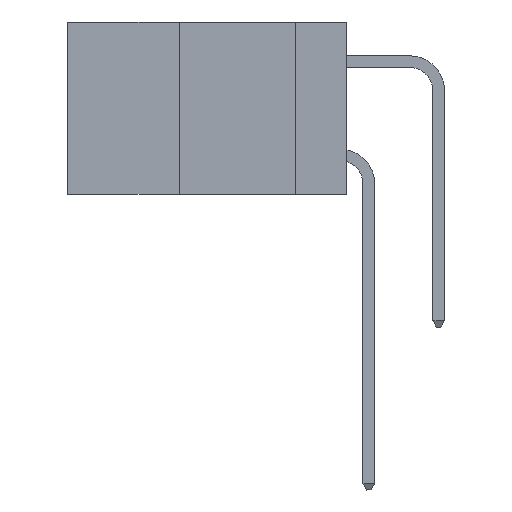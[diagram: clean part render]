
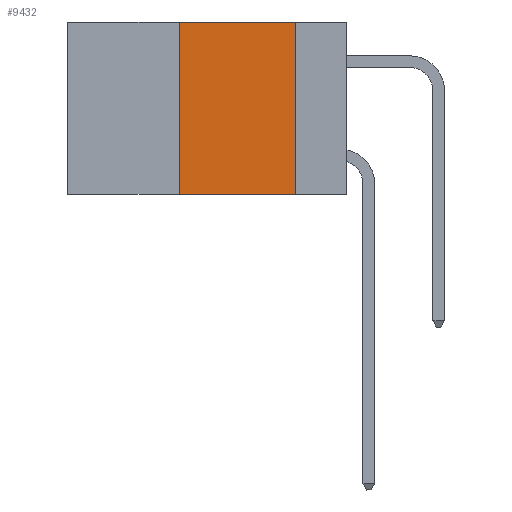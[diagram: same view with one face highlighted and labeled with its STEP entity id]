
A CAD part, left-side view. The second image highlights one B-rep face of the part: STEP entity #9432.
In plain terms, the highlighted planar face has unit normal (-1, 0, 0).
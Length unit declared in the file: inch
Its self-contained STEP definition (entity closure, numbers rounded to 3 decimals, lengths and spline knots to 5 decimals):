
#550 = LINE ( 'NONE', #8312, #8073 ) ;
#907 = ORIENTED_EDGE ( 'NONE', *, *, #11543, .F. ) ;
#1403 = LINE ( 'NONE', #4061, #6314 ) ;
#1874 = CARTESIAN_POINT ( 'NONE',  ( 0., 0.11, -0.37 ) ) ;
#1982 = CARTESIAN_POINT ( 'NONE',  ( 0., 0.36, -0.37 ) ) ;
#2194 = CARTESIAN_POINT ( 'NONE',  ( 0., 0.11, 0. ) ) ;
#2988 = LINE ( 'NONE', #5645, #7509 ) ;
#3065 = VERTEX_POINT ( 'NONE', #3408 ) ;
#3408 = CARTESIAN_POINT ( 'NONE',  ( 0., 0.36, 0. ) ) ;
#3437 = DIRECTION ( 'NONE',  ( 1., 0., 0. ) ) ;
#3936 = ORIENTED_EDGE ( 'NONE', *, *, #5729, .F. ) ;
#4061 = CARTESIAN_POINT ( 'NONE',  ( 0., 0.11, 0. ) ) ;
#4107 = DIRECTION ( 'NONE',  ( 0., 0., -1. ) ) ;
#4179 = LINE ( 'NONE', #4275, #7334 ) ;
#4275 = CARTESIAN_POINT ( 'NONE',  ( 0., 0.36, 0. ) ) ;
#4535 = EDGE_CURVE ( 'NONE', #11999, #9100, #2988, .T. ) ;
#4702 = ORIENTED_EDGE ( 'NONE', *, *, #4535, .T. ) ;
#5645 = CARTESIAN_POINT ( 'NONE',  ( 0., 0.6, -0.37 ) ) ;
#5729 = EDGE_CURVE ( 'NONE', #12109, #9100, #1403, .T. ) ;
#6010 = FACE_OUTER_BOUND ( 'NONE', #9294, .T. ) ;
#6205 = AXIS2_PLACEMENT_3D ( 'NONE', #8195, #3437, #10033 ) ;
#6314 = VECTOR ( 'NONE', #4107, 39.37008 ) ;
#6315 = PLANE ( 'NONE',  #6205 ) ;
#7334 = VECTOR ( 'NONE', #10843, 39.37008 ) ;
#7509 = VECTOR ( 'NONE', #11250, 39.37008 ) ;
#8073 = VECTOR ( 'NONE', #11093, 39.37008 ) ;
#8195 = CARTESIAN_POINT ( 'NONE',  ( 0., 0.6, 0. ) ) ;
#8312 = CARTESIAN_POINT ( 'NONE',  ( 0., 0.6, 0. ) ) ;
#8667 = ORIENTED_EDGE ( 'NONE', *, *, #10124, .F. ) ;
#9100 = VERTEX_POINT ( 'NONE', #1874 ) ;
#9294 = EDGE_LOOP ( 'NONE', ( #3936, #8667, #907, #4702 ) ) ;
#9432 = ADVANCED_FACE ( 'NONE', ( #6010 ), #6315, .F. ) ;
#10033 = DIRECTION ( 'NONE',  ( 0., 0., -1. ) ) ;
#10124 = EDGE_CURVE ( 'NONE', #3065, #12109, #550, .T. ) ;
#10843 = DIRECTION ( 'NONE',  ( 0., 0., 1. ) ) ;
#11093 = DIRECTION ( 'NONE',  ( 0., -1., 0. ) ) ;
#11250 = DIRECTION ( 'NONE',  ( 0., -1., 0. ) ) ;
#11543 = EDGE_CURVE ( 'NONE', #11999, #3065, #4179, .T. ) ;
#11999 = VERTEX_POINT ( 'NONE', #1982 ) ;
#12109 = VERTEX_POINT ( 'NONE', #2194 ) ;
